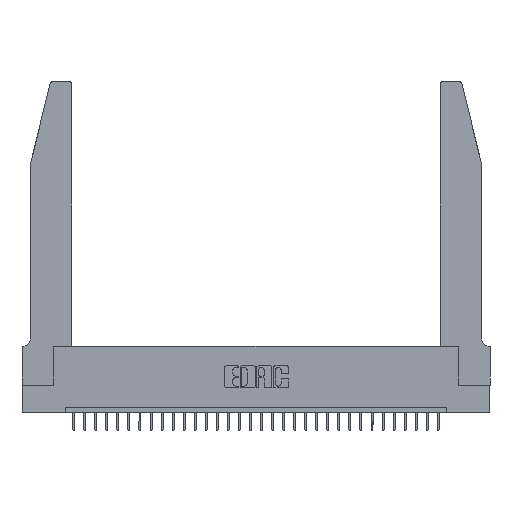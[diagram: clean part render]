
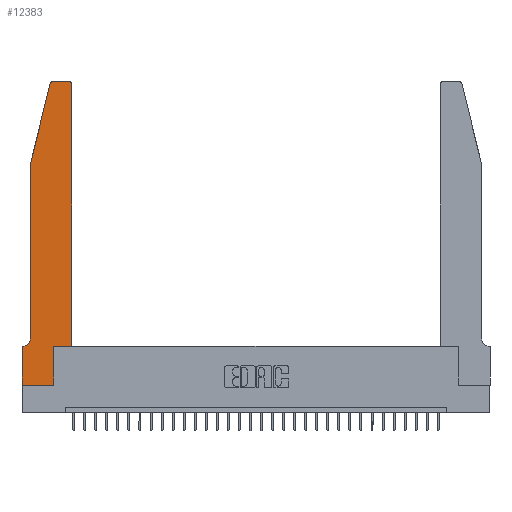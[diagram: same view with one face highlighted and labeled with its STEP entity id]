
A CAD part, top view. The second image highlights one B-rep face of the part: STEP entity #12383.
In plain terms, the highlighted planar face has unit normal (0, 0, 1).
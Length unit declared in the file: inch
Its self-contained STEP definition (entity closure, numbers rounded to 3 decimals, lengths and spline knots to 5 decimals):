
#468 = LINE ( 'NONE', #18030, #8375 ) ;
#498 = AXIS2_PLACEMENT_3D ( 'NONE', #13550, #11075, #15779 ) ;
#577 = FACE_OUTER_BOUND ( 'NONE', #3819, .T. ) ;
#739 = ORIENTED_EDGE ( 'NONE', *, *, #15765, .T. ) ;
#1134 = DIRECTION ( 'NONE',  ( 1., 0., 0. ) ) ;
#1259 = CIRCLE ( 'NONE', #5562, 0.07 ) ;
#1297 = CARTESIAN_POINT ( 'NONE',  ( 0.284, 2.75, 0.37 ) ) ;
#2380 = VECTOR ( 'NONE', #21651, 39.37008 ) ;
#2996 = VECTOR ( 'NONE', #26868, 39.37008 ) ;
#3321 = ORIENTED_EDGE ( 'NONE', *, *, #9594, .T. ) ;
#3374 = EDGE_CURVE ( 'NONE', #23425, #17346, #1259, .T. ) ;
#3799 = VERTEX_POINT ( 'NONE', #24970 ) ;
#3819 = EDGE_LOOP ( 'NONE', ( #19563, #26219, #30710, #23294, #12534, #9690, #13311, #7512, #3321, #739, #23184, #10381 ) ) ;
#4358 = DIRECTION ( 'NONE',  ( 1., 0., 0. ) ) ;
#5562 = AXIS2_PLACEMENT_3D ( 'NONE', #27044, #20088, #15110 ) ;
#6069 = CARTESIAN_POINT ( 'NONE',  ( 0.4205, 2.72, 0.37 ) ) ;
#7030 = VERTEX_POINT ( 'NONE', #1297 ) ;
#7426 = CARTESIAN_POINT ( 'NONE',  ( 0.0055, 0.35, 0.37 ) ) ;
#7512 = ORIENTED_EDGE ( 'NONE', *, *, #7518, .T. ) ;
#7518 = EDGE_CURVE ( 'NONE', #10493, #18581, #468, .T. ) ;
#7619 = VERTEX_POINT ( 'NONE', #23140 ) ;
#8025 = CARTESIAN_POINT ( 'NONE',  ( 0., 0., 0.37 ) ) ;
#8096 = EDGE_CURVE ( 'NONE', #24509, #7030, #30488, .T. ) ;
#8211 = DIRECTION ( 'NONE',  ( 0., 0., 1. ) ) ;
#8264 = VECTOR ( 'NONE', #10169, 39.37008 ) ;
#8375 = VECTOR ( 'NONE', #15403, 39.37008 ) ;
#8506 = EDGE_CURVE ( 'NONE', #17346, #26343, #11815, .T. ) ;
#8642 = PLANE ( 'NONE',  #22774 ) ;
#9525 = CARTESIAN_POINT ( 'NONE',  ( 0.0755, 2., 0.37 ) ) ;
#9594 = EDGE_CURVE ( 'NONE', #18581, #3799, #12489, .T. ) ;
#9690 = ORIENTED_EDGE ( 'NONE', *, *, #8506, .T. ) ;
#10169 = DIRECTION ( 'NONE',  ( 0., 1., 0. ) ) ;
#10213 = EDGE_CURVE ( 'NONE', #13896, #24509, #10549, .T. ) ;
#10381 = ORIENTED_EDGE ( 'NONE', *, *, #10213, .T. ) ;
#10493 = VERTEX_POINT ( 'NONE', #12582 ) ;
#10549 = CIRCLE ( 'NONE', #22148, 0.03 ) ;
#10893 = VECTOR ( 'NONE', #11992, 39.37008 ) ;
#11075 = DIRECTION ( 'NONE',  ( 0., 0., 1. ) ) ;
#11718 = EDGE_CURVE ( 'NONE', #26343, #10493, #16121, .T. ) ;
#11815 = LINE ( 'NONE', #12847, #29722 ) ;
#11992 = DIRECTION ( 'NONE',  ( -0.239, -0.971, 0. ) ) ;
#12383 = ADVANCED_FACE ( 'NONE', ( #577 ), #8642, .T. ) ;
#12489 = LINE ( 'NONE', #25004, #8264 ) ;
#12534 = ORIENTED_EDGE ( 'NONE', *, *, #3374, .T. ) ;
#12582 = CARTESIAN_POINT ( 'NONE',  ( 0., 0., 0.37 ) ) ;
#12847 = CARTESIAN_POINT ( 'NONE',  ( 0.0755, 0.35, 0.37 ) ) ;
#12919 = CARTESIAN_POINT ( 'NONE',  ( 0., 0.35, 0.37 ) ) ;
#13012 = CARTESIAN_POINT ( 'NONE',  ( 0.2865, 0., 0.37 ) ) ;
#13040 = CARTESIAN_POINT ( 'NONE',  ( 0.25487, 2.72718, 0.37 ) ) ;
#13311 = ORIENTED_EDGE ( 'NONE', *, *, #11718, .T. ) ;
#13550 = CARTESIAN_POINT ( 'NONE',  ( 0.284, 2.72, 0.37 ) ) ;
#13896 = VERTEX_POINT ( 'NONE', #16053 ) ;
#14385 = VECTOR ( 'NONE', #4358, 39.37008 ) ;
#15019 = CIRCLE ( 'NONE', #498, 0.03 ) ;
#15110 = DIRECTION ( 'NONE',  ( -1., 0., 0. ) ) ;
#15159 = VERTEX_POINT ( 'NONE', #23541 ) ;
#15316 = EDGE_CURVE ( 'NONE', #15159, #13896, #15912, .T. ) ;
#15403 = DIRECTION ( 'NONE',  ( 1., 0., 0. ) ) ;
#15599 = DIRECTION ( 'NONE',  ( -1., 0., 0. ) ) ;
#15765 = EDGE_CURVE ( 'NONE', #3799, #15159, #23106, .T. ) ;
#15779 = DIRECTION ( 'NONE',  ( 1., 0., 0. ) ) ;
#15912 = LINE ( 'NONE', #19383, #2996 ) ;
#16053 = CARTESIAN_POINT ( 'NONE',  ( 0.4505, 2.72, 0.37 ) ) ;
#16121 = LINE ( 'NONE', #8025, #24181 ) ;
#16190 = EDGE_CURVE ( 'NONE', #22086, #7619, #19676, .T. ) ;
#17346 = VERTEX_POINT ( 'NONE', #7426 ) ;
#18030 = CARTESIAN_POINT ( 'NONE',  ( 0., 0., 0.37 ) ) ;
#18213 = EDGE_CURVE ( 'NONE', #7030, #22086, #15019, .T. ) ;
#18581 = VERTEX_POINT ( 'NONE', #13012 ) ;
#18967 = CARTESIAN_POINT ( 'NONE',  ( 0.0755, 2., 0.37 ) ) ;
#19383 = CARTESIAN_POINT ( 'NONE',  ( 0.4505, 0.35, 0.37 ) ) ;
#19563 = ORIENTED_EDGE ( 'NONE', *, *, #8096, .T. ) ;
#19676 = LINE ( 'NONE', #9525, #10893 ) ;
#20088 = DIRECTION ( 'NONE',  ( 0., 0., -1. ) ) ;
#20336 = EDGE_CURVE ( 'NONE', #7619, #23425, #22882, .T. ) ;
#21651 = DIRECTION ( 'NONE',  ( 0., -1., 0. ) ) ;
#22086 = VERTEX_POINT ( 'NONE', #13040 ) ;
#22148 = AXIS2_PLACEMENT_3D ( 'NONE', #6069, #8211, #1134 ) ;
#22774 = AXIS2_PLACEMENT_3D ( 'NONE', #25931, #25725, #30595 ) ;
#22882 = LINE ( 'NONE', #18967, #2380 ) ;
#23106 = LINE ( 'NONE', #26195, #14385 ) ;
#23140 = CARTESIAN_POINT ( 'NONE',  ( 0.0755, 2., 0.37 ) ) ;
#23184 = ORIENTED_EDGE ( 'NONE', *, *, #15316, .T. ) ;
#23281 = CARTESIAN_POINT ( 'NONE',  ( 0.4205, 2.75, 0.37 ) ) ;
#23294 = ORIENTED_EDGE ( 'NONE', *, *, #20336, .T. ) ;
#23425 = VERTEX_POINT ( 'NONE', #28625 ) ;
#23541 = CARTESIAN_POINT ( 'NONE',  ( 0.4505, 0.35, 0.37 ) ) ;
#24181 = VECTOR ( 'NONE', #27553, 39.37008 ) ;
#24509 = VERTEX_POINT ( 'NONE', #23281 ) ;
#24970 = CARTESIAN_POINT ( 'NONE',  ( 0.2865, 0.35, 0.37 ) ) ;
#25004 = CARTESIAN_POINT ( 'NONE',  ( 0.2865, 0.35, 0.37 ) ) ;
#25725 = DIRECTION ( 'NONE',  ( 0., 0., 1. ) ) ;
#25930 = VECTOR ( 'NONE', #29104, 39.37008 ) ;
#25931 = CARTESIAN_POINT ( 'NONE',  ( 0., 0.35, 0.37 ) ) ;
#26195 = CARTESIAN_POINT ( 'NONE',  ( 0.4505, 0.35, 0.37 ) ) ;
#26219 = ORIENTED_EDGE ( 'NONE', *, *, #18213, .T. ) ;
#26343 = VERTEX_POINT ( 'NONE', #12919 ) ;
#26868 = DIRECTION ( 'NONE',  ( 0., 1., 0. ) ) ;
#27044 = CARTESIAN_POINT ( 'NONE',  ( 0.0055, 0.42, 0.37 ) ) ;
#27553 = DIRECTION ( 'NONE',  ( 0., -1., 0. ) ) ;
#28625 = CARTESIAN_POINT ( 'NONE',  ( 0.0755, 0.42, 0.37 ) ) ;
#29104 = DIRECTION ( 'NONE',  ( -1., 0., 0. ) ) ;
#29416 = CARTESIAN_POINT ( 'NONE',  ( 0.2605, 2.75, 0.37 ) ) ;
#29722 = VECTOR ( 'NONE', #15599, 39.37008 ) ;
#30488 = LINE ( 'NONE', #29416, #25930 ) ;
#30595 = DIRECTION ( 'NONE',  ( 1., 0., 0. ) ) ;
#30710 = ORIENTED_EDGE ( 'NONE', *, *, #16190, .T. ) ;
